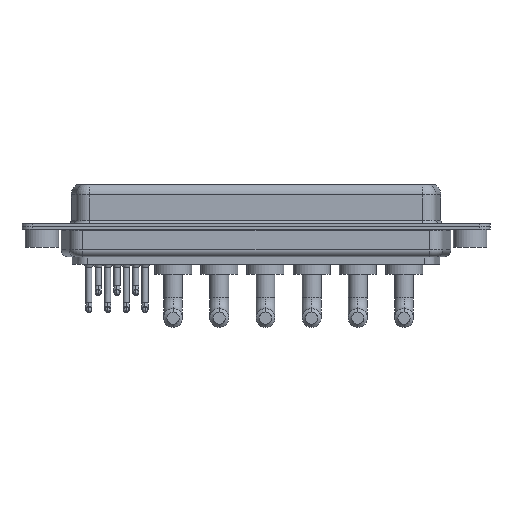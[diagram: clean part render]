
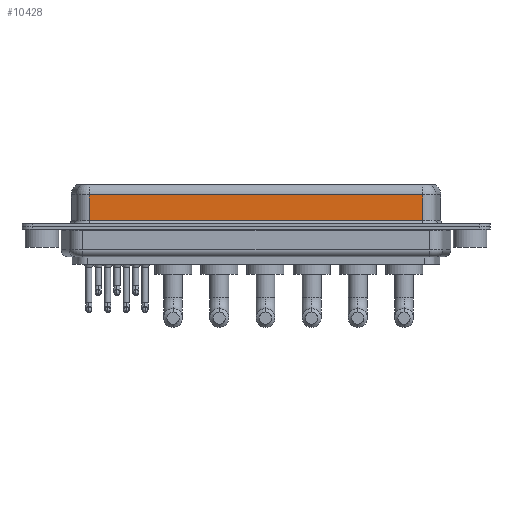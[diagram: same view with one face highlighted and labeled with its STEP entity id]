
A CAD part, front view. The second image highlights one B-rep face of the part: STEP entity #10428.
In plain terms, the highlighted planar face has unit normal (0, -1, 0).
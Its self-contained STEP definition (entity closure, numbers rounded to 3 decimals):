
#228 = VECTOR ( 'NONE', #16304, 1000. ) ;
#327 = CARTESIAN_POINT ( 'NONE',  ( 56.462, -3.95, 0.9 ) ) ;
#1575 = EDGE_CURVE ( 'NONE', #17529, #3818, #6373, .T. ) ;
#1668 = PLANE ( 'NONE',  #11938 ) ;
#1763 = CARTESIAN_POINT ( 'NONE',  ( 56.462, -3.95, 4.65 ) ) ;
#1865 = ORIENTED_EDGE ( 'NONE', *, *, #10290, .T. ) ;
#2342 = ORIENTED_EDGE ( 'NONE', *, *, #7210, .T. ) ;
#3335 = DIRECTION ( 'NONE',  ( 0., 0., 1. ) ) ;
#3653 = ORIENTED_EDGE ( 'NONE', *, *, #14511, .T. ) ;
#3818 = VERTEX_POINT ( 'NONE', #327 ) ;
#4052 = LINE ( 'NONE', #8158, #6046 ) ;
#4790 = ORIENTED_EDGE ( 'NONE', *, *, #1575, .F. ) ;
#4829 = CARTESIAN_POINT ( 'NONE',  ( 56.462, -3.95, 4.65 ) ) ;
#4904 = CARTESIAN_POINT ( 'NONE',  ( 56.462, -3.95, 6.4 ) ) ;
#5008 = CARTESIAN_POINT ( 'NONE',  ( 7.038, -3.95, 0.9 ) ) ;
#6046 = VECTOR ( 'NONE', #6748, 1000. ) ;
#6373 = LINE ( 'NONE', #4904, #17743 ) ;
#6748 = DIRECTION ( 'NONE',  ( 1., 0., 0. ) ) ;
#7210 = EDGE_CURVE ( 'NONE', #16539, #9111, #15261, .T. ) ;
#7947 = CARTESIAN_POINT ( 'NONE',  ( 7.038, -3.95, 4.65 ) ) ;
#8149 = CARTESIAN_POINT ( 'NONE',  ( 7.038, -3.95, 6.4 ) ) ;
#8158 = CARTESIAN_POINT ( 'NONE',  ( 56.462, -3.95, 0.9 ) ) ;
#9111 = VERTEX_POINT ( 'NONE', #5008 ) ;
#10290 = EDGE_CURVE ( 'NONE', #17529, #16539, #15497, .T. ) ;
#10428 = ADVANCED_FACE ( 'NONE', ( #10437 ), #1668, .F. ) ;
#10437 = FACE_OUTER_BOUND ( 'NONE', #18411, .T. ) ;
#10602 = DIRECTION ( 'NONE',  ( 0., 0., -1. ) ) ;
#11632 = VECTOR ( 'NONE', #13320, 1000. ) ;
#11938 = AXIS2_PLACEMENT_3D ( 'NONE', #13036, #16134, #3335 ) ;
#13036 = CARTESIAN_POINT ( 'NONE',  ( 56.462, -3.95, 6.4 ) ) ;
#13320 = DIRECTION ( 'NONE',  ( -1., 0., 0. ) ) ;
#14511 = EDGE_CURVE ( 'NONE', #9111, #3818, #4052, .T. ) ;
#15261 = LINE ( 'NONE', #8149, #228 ) ;
#15497 = LINE ( 'NONE', #1763, #11632 ) ;
#16134 = DIRECTION ( 'NONE',  ( 0., 1., 0. ) ) ;
#16304 = DIRECTION ( 'NONE',  ( 0., 0., -1. ) ) ;
#16539 = VERTEX_POINT ( 'NONE', #7947 ) ;
#17529 = VERTEX_POINT ( 'NONE', #4829 ) ;
#17743 = VECTOR ( 'NONE', #10602, 1000. ) ;
#18411 = EDGE_LOOP ( 'NONE', ( #4790, #1865, #2342, #3653 ) ) ;
